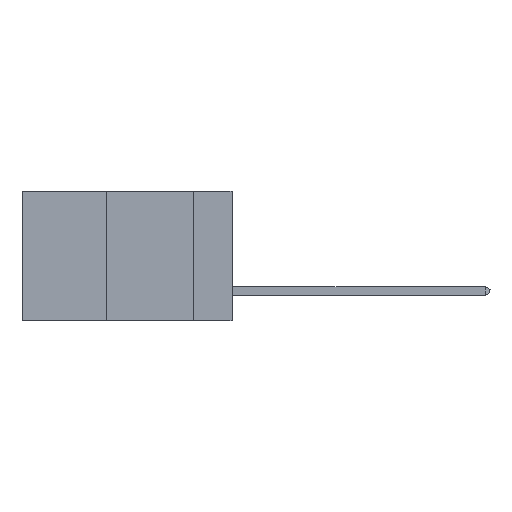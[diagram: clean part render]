
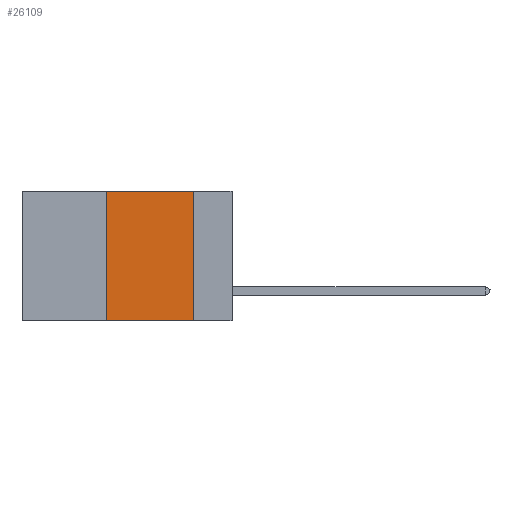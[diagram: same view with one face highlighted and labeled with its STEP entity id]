
A CAD part, left-side view. The second image highlights one B-rep face of the part: STEP entity #26109.
In plain terms, the highlighted planar face has unit normal (-1, 0, 0).
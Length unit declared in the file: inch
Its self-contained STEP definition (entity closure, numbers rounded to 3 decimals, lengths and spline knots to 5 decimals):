
#364 = VERTEX_POINT ( 'NONE', #4419 ) ;
#730 = DIRECTION ( 'NONE',  ( 0., -1., 0. ) ) ;
#2416 = DIRECTION ( 'NONE',  ( 0., -1., 0. ) ) ;
#2607 = FACE_OUTER_BOUND ( 'NONE', #12451, .T. ) ;
#3951 = LINE ( 'NONE', #38416, #18443 ) ;
#4419 = CARTESIAN_POINT ( 'NONE',  ( 0., 0.36, 0. ) ) ;
#5834 = CARTESIAN_POINT ( 'NONE',  ( 0., 0.6, -0.37 ) ) ;
#6020 = CARTESIAN_POINT ( 'NONE',  ( 0., 0.11, 0. ) ) ;
#6594 = DIRECTION ( 'NONE',  ( 0., 0., -1. ) ) ;
#6596 = AXIS2_PLACEMENT_3D ( 'NONE', #31910, #13288, #6594 ) ;
#7796 = LINE ( 'NONE', #24049, #31536 ) ;
#10403 = ORIENTED_EDGE ( 'NONE', *, *, #27832, .F. ) ;
#11517 = VECTOR ( 'NONE', #13070, 39.37008 ) ;
#11874 = CARTESIAN_POINT ( 'NONE',  ( 0., 0.36, -0.37 ) ) ;
#12451 = EDGE_LOOP ( 'NONE', ( #10403, #30740, #33174, #37633 ) ) ;
#13070 = DIRECTION ( 'NONE',  ( 0., 0., 1. ) ) ;
#13288 = DIRECTION ( 'NONE',  ( 1., 0., 0. ) ) ;
#13545 = EDGE_CURVE ( 'NONE', #364, #24063, #3951, .T. ) ;
#13608 = VECTOR ( 'NONE', #2416, 39.37008 ) ;
#18443 = VECTOR ( 'NONE', #730, 39.37008 ) ;
#24049 = CARTESIAN_POINT ( 'NONE',  ( 0., 0.11, 0. ) ) ;
#24063 = VERTEX_POINT ( 'NONE', #6020 ) ;
#25880 = VERTEX_POINT ( 'NONE', #11874 ) ;
#26109 = ADVANCED_FACE ( 'NONE', ( #2607 ), #31775, .F. ) ;
#26426 = VERTEX_POINT ( 'NONE', #30001 ) ;
#26721 = LINE ( 'NONE', #5834, #13608 ) ;
#27832 = EDGE_CURVE ( 'NONE', #24063, #26426, #7796, .T. ) ;
#29175 = EDGE_CURVE ( 'NONE', #25880, #364, #31401, .T. ) ;
#30001 = CARTESIAN_POINT ( 'NONE',  ( 0., 0.11, -0.37 ) ) ;
#30740 = ORIENTED_EDGE ( 'NONE', *, *, #13545, .F. ) ;
#31401 = LINE ( 'NONE', #34428, #11517 ) ;
#31536 = VECTOR ( 'NONE', #36311, 39.37008 ) ;
#31775 = PLANE ( 'NONE',  #6596 ) ;
#31910 = CARTESIAN_POINT ( 'NONE',  ( 0., 0.6, 0. ) ) ;
#33174 = ORIENTED_EDGE ( 'NONE', *, *, #29175, .F. ) ;
#33602 = EDGE_CURVE ( 'NONE', #25880, #26426, #26721, .T. ) ;
#34428 = CARTESIAN_POINT ( 'NONE',  ( 0., 0.36, 0. ) ) ;
#36311 = DIRECTION ( 'NONE',  ( 0., 0., -1. ) ) ;
#37633 = ORIENTED_EDGE ( 'NONE', *, *, #33602, .T. ) ;
#38416 = CARTESIAN_POINT ( 'NONE',  ( 0., 0.6, 0. ) ) ;
